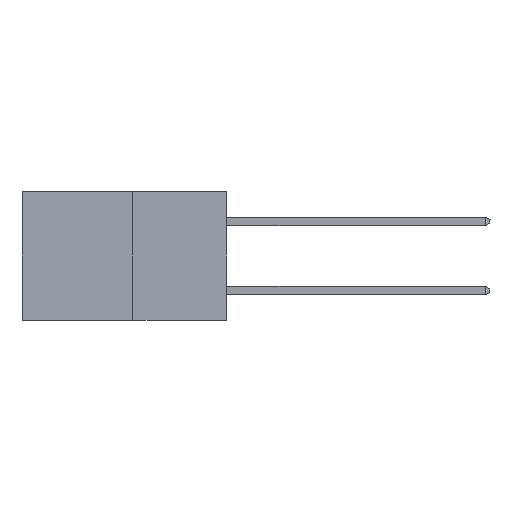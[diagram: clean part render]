
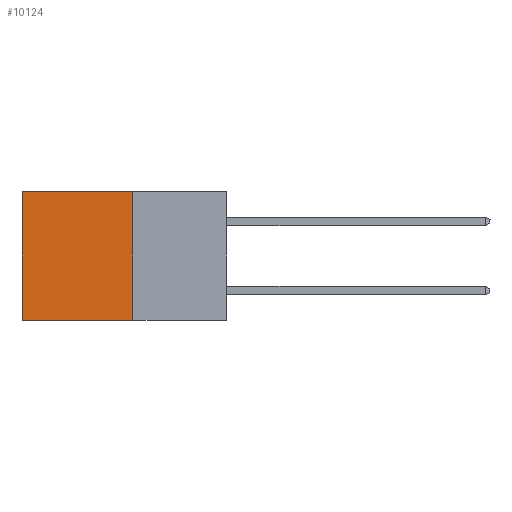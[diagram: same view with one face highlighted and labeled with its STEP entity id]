
A CAD part, left-side view. The second image highlights one B-rep face of the part: STEP entity #10124.
In plain terms, the highlighted planar face has unit normal (-1, 0, 0).
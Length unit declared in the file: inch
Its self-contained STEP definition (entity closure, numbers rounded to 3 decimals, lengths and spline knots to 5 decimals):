
#1444 = CARTESIAN_POINT ( 'NONE',  ( 0.277, 0.27, -0.37 ) ) ;
#1730 = CARTESIAN_POINT ( 'NONE',  ( 0.277, 0.59, -0.37 ) ) ;
#2051 = LINE ( 'NONE', #3473, #14330 ) ;
#2847 = LINE ( 'NONE', #9455, #6845 ) ;
#3473 = CARTESIAN_POINT ( 'NONE',  ( 0.277, 0.27, -0.37 ) ) ;
#3847 = AXIS2_PLACEMENT_3D ( 'NONE', #7058, #8700, #20117 ) ;
#5350 = PLANE ( 'NONE',  #3847 ) ;
#5858 = ORIENTED_EDGE ( 'NONE', *, *, #17159, .F. ) ;
#6845 = VECTOR ( 'NONE', #14437, 39.37008 ) ;
#7058 = CARTESIAN_POINT ( 'NONE',  ( 0.277, 0.27, -0.37 ) ) ;
#8052 = VERTEX_POINT ( 'NONE', #20290 ) ;
#8424 = VECTOR ( 'NONE', #18875, 39.37008 ) ;
#8464 = DIRECTION ( 'NONE',  ( 0., 0., -1. ) ) ;
#8473 = EDGE_LOOP ( 'NONE', ( #19731, #5858, #13223, #13260 ) ) ;
#8700 = DIRECTION ( 'NONE',  ( 1., 0., 0. ) ) ;
#9455 = CARTESIAN_POINT ( 'NONE',  ( 0.277, 0.27, 0. ) ) ;
#10124 = ADVANCED_FACE ( 'NONE', ( #20923 ), #5350, .F. ) ;
#12519 = VECTOR ( 'NONE', #16319, 39.37008 ) ;
#12747 = EDGE_CURVE ( 'NONE', #12811, #17718, #2051, .T. ) ;
#12811 = VERTEX_POINT ( 'NONE', #20093 ) ;
#13037 = LINE ( 'NONE', #1444, #12519 ) ;
#13223 = ORIENTED_EDGE ( 'NONE', *, *, #12747, .F. ) ;
#13260 = ORIENTED_EDGE ( 'NONE', *, *, #17010, .T. ) ;
#14330 = VECTOR ( 'NONE', #8464, 39.37008 ) ;
#14437 = DIRECTION ( 'NONE',  ( 0., 1., 0. ) ) ;
#14693 = CARTESIAN_POINT ( 'NONE',  ( 0.277, 0.27, -0.37 ) ) ;
#16092 = EDGE_CURVE ( 'NONE', #8052, #17293, #16645, .T. ) ;
#16319 = DIRECTION ( 'NONE',  ( 0., 1., 0. ) ) ;
#16645 = LINE ( 'NONE', #17224, #8424 ) ;
#17010 = EDGE_CURVE ( 'NONE', #12811, #8052, #2847, .T. ) ;
#17159 = EDGE_CURVE ( 'NONE', #17718, #17293, #13037, .T. ) ;
#17224 = CARTESIAN_POINT ( 'NONE',  ( 0.277, 0.59, -0.37 ) ) ;
#17293 = VERTEX_POINT ( 'NONE', #1730 ) ;
#17718 = VERTEX_POINT ( 'NONE', #14693 ) ;
#18875 = DIRECTION ( 'NONE',  ( 0., 0., -1. ) ) ;
#19731 = ORIENTED_EDGE ( 'NONE', *, *, #16092, .T. ) ;
#20093 = CARTESIAN_POINT ( 'NONE',  ( 0.277, 0.27, 0. ) ) ;
#20117 = DIRECTION ( 'NONE',  ( 0., 0., -1. ) ) ;
#20290 = CARTESIAN_POINT ( 'NONE',  ( 0.277, 0.59, 0. ) ) ;
#20923 = FACE_OUTER_BOUND ( 'NONE', #8473, .T. ) ;
